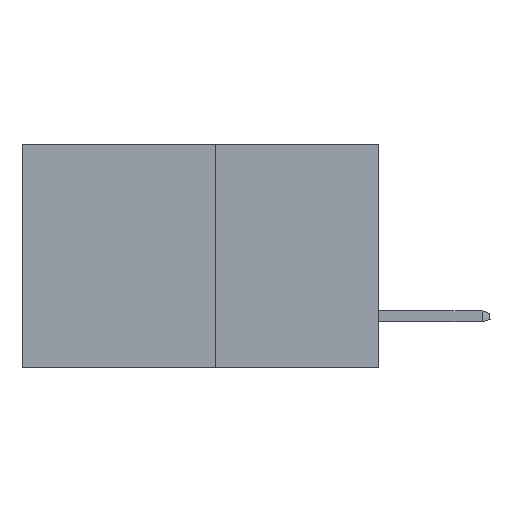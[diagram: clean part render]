
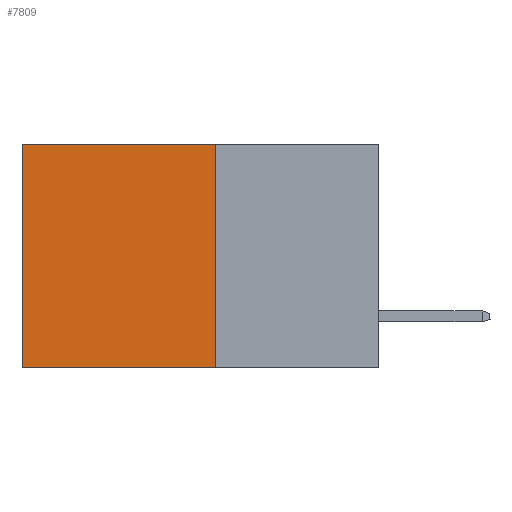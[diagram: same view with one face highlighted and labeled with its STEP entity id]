
A CAD part, left-side view. The second image highlights one B-rep face of the part: STEP entity #7809.
In plain terms, the highlighted planar face has unit normal (-1, 0, 0).
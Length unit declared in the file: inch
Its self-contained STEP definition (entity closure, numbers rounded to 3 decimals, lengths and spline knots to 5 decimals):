
#428 = LINE ( 'NONE', #1702, #6554 ) ;
#605 = LINE ( 'NONE', #4665, #17915 ) ;
#1423 = LINE ( 'NONE', #7390, #13874 ) ;
#1602 = VERTEX_POINT ( 'NONE', #14891 ) ;
#1702 = CARTESIAN_POINT ( 'NONE',  ( 0.277, 0.27, 0. ) ) ;
#4159 = CARTESIAN_POINT ( 'NONE',  ( 0.277, 0.59, -0.37 ) ) ;
#4374 = ORIENTED_EDGE ( 'NONE', *, *, #11334, .T. ) ;
#4665 = CARTESIAN_POINT ( 'NONE',  ( 0.277, 0.59, -0.37 ) ) ;
#5642 = CARTESIAN_POINT ( 'NONE',  ( 0.277, 0.27, -0.37 ) ) ;
#5683 = ORIENTED_EDGE ( 'NONE', *, *, #19931, .F. ) ;
#6554 = VECTOR ( 'NONE', #18503, 39.37008 ) ;
#6726 = ORIENTED_EDGE ( 'NONE', *, *, #7850, .F. ) ;
#7010 = VERTEX_POINT ( 'NONE', #4159 ) ;
#7317 = DIRECTION ( 'NONE',  ( 1., 0., 0. ) ) ;
#7390 = CARTESIAN_POINT ( 'NONE',  ( 0.277, 0.27, -0.37 ) ) ;
#7809 = ADVANCED_FACE ( 'NONE', ( #10975 ), #15633, .F. ) ;
#7850 = EDGE_CURVE ( 'NONE', #18965, #16480, #1423, .T. ) ;
#9094 = DIRECTION ( 'NONE',  ( 0., 0., -1. ) ) ;
#10286 = AXIS2_PLACEMENT_3D ( 'NONE', #5642, #7317, #18994 ) ;
#10975 = FACE_OUTER_BOUND ( 'NONE', #16242, .T. ) ;
#11334 = EDGE_CURVE ( 'NONE', #18965, #1602, #428, .T. ) ;
#11399 = DIRECTION ( 'NONE',  ( 0., 0., -1. ) ) ;
#12834 = CARTESIAN_POINT ( 'NONE',  ( 0.277, 0.27, -0.37 ) ) ;
#13264 = CARTESIAN_POINT ( 'NONE',  ( 0.277, 0.27, 0. ) ) ;
#13874 = VECTOR ( 'NONE', #9094, 39.37008 ) ;
#13954 = EDGE_CURVE ( 'NONE', #1602, #7010, #605, .T. ) ;
#14891 = CARTESIAN_POINT ( 'NONE',  ( 0.277, 0.59, 0. ) ) ;
#15633 = PLANE ( 'NONE',  #10286 ) ;
#16242 = EDGE_LOOP ( 'NONE', ( #18462, #5683, #6726, #4374 ) ) ;
#16480 = VERTEX_POINT ( 'NONE', #16572 ) ;
#16572 = CARTESIAN_POINT ( 'NONE',  ( 0.277, 0.27, -0.37 ) ) ;
#16789 = VECTOR ( 'NONE', #17761, 39.37008 ) ;
#17761 = DIRECTION ( 'NONE',  ( 0., 1., 0. ) ) ;
#17915 = VECTOR ( 'NONE', #11399, 39.37008 ) ;
#18462 = ORIENTED_EDGE ( 'NONE', *, *, #13954, .T. ) ;
#18503 = DIRECTION ( 'NONE',  ( 0., 1., 0. ) ) ;
#18965 = VERTEX_POINT ( 'NONE', #13264 ) ;
#18994 = DIRECTION ( 'NONE',  ( 0., 0., -1. ) ) ;
#19931 = EDGE_CURVE ( 'NONE', #16480, #7010, #21234, .T. ) ;
#21234 = LINE ( 'NONE', #12834, #16789 ) ;
